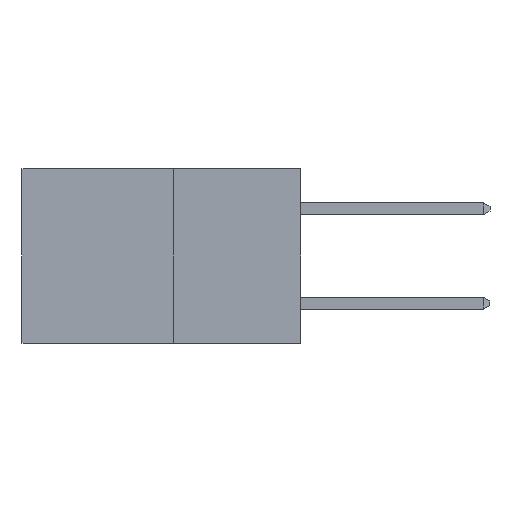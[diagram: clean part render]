
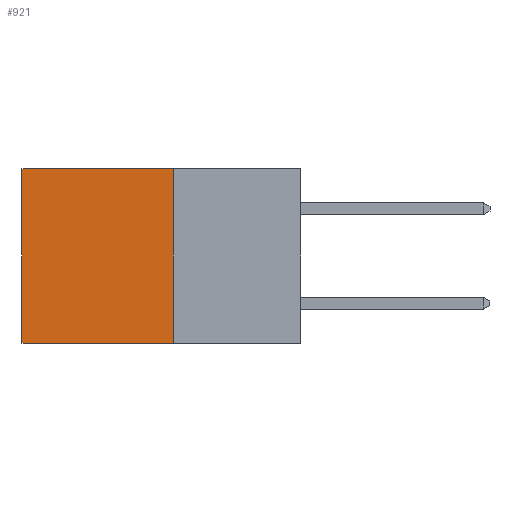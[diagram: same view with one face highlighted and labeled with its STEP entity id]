
A CAD part, left-side view. The second image highlights one B-rep face of the part: STEP entity #921.
In plain terms, the highlighted planar face has unit normal (-1, 0, 0).
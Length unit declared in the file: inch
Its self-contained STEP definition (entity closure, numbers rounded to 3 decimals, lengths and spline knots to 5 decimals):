
#343 = CARTESIAN_POINT ( 'NONE',  ( 0.277, 0.27, -0.37 ) ) ;
#373 = EDGE_LOOP ( 'NONE', ( #2014, #1810, #726, #1979 ) ) ;
#726 = ORIENTED_EDGE ( 'NONE', *, *, #4513, .F. ) ;
#759 = CARTESIAN_POINT ( 'NONE',  ( 0.277, 0.27, -0.37 ) ) ;
#921 = ADVANCED_FACE ( 'NONE', ( #6134 ), #6779, .F. ) ;
#927 = VERTEX_POINT ( 'NONE', #343 ) ;
#1200 = EDGE_CURVE ( 'NONE', #4449, #5701, #6830, .T. ) ;
#1810 = ORIENTED_EDGE ( 'NONE', *, *, #2150, .F. ) ;
#1979 = ORIENTED_EDGE ( 'NONE', *, *, #7679, .T. ) ;
#2014 = ORIENTED_EDGE ( 'NONE', *, *, #1200, .T. ) ;
#2150 = EDGE_CURVE ( 'NONE', #927, #5701, #4479, .T. ) ;
#3275 = VECTOR ( 'NONE', #7801, 39.37008 ) ;
#3278 = CARTESIAN_POINT ( 'NONE',  ( 0.277, 0.59, 0. ) ) ;
#3929 = VECTOR ( 'NONE', #7416, 39.37008 ) ;
#4286 = VECTOR ( 'NONE', #6316, 39.37008 ) ;
#4449 = VERTEX_POINT ( 'NONE', #3278 ) ;
#4478 = LINE ( 'NONE', #6309, #4286 ) ;
#4479 = LINE ( 'NONE', #5652, #3275 ) ;
#4513 = EDGE_CURVE ( 'NONE', #7478, #927, #4478, .T. ) ;
#4725 = DIRECTION ( 'NONE',  ( 1., 0., 0. ) ) ;
#4797 = VECTOR ( 'NONE', #7681, 39.37008 ) ;
#4952 = CARTESIAN_POINT ( 'NONE',  ( 0.277, 0.27, 0. ) ) ;
#5436 = DIRECTION ( 'NONE',  ( 0., 0., -1. ) ) ;
#5652 = CARTESIAN_POINT ( 'NONE',  ( 0.277, 0.27, -0.37 ) ) ;
#5701 = VERTEX_POINT ( 'NONE', #6427 ) ;
#6134 = FACE_OUTER_BOUND ( 'NONE', #373, .T. ) ;
#6309 = CARTESIAN_POINT ( 'NONE',  ( 0.277, 0.27, -0.37 ) ) ;
#6316 = DIRECTION ( 'NONE',  ( 0., 0., -1. ) ) ;
#6351 = LINE ( 'NONE', #7615, #4797 ) ;
#6427 = CARTESIAN_POINT ( 'NONE',  ( 0.277, 0.59, -0.37 ) ) ;
#6779 = PLANE ( 'NONE',  #7585 ) ;
#6830 = LINE ( 'NONE', #6902, #3929 ) ;
#6902 = CARTESIAN_POINT ( 'NONE',  ( 0.277, 0.59, -0.37 ) ) ;
#7416 = DIRECTION ( 'NONE',  ( 0., 0., -1. ) ) ;
#7478 = VERTEX_POINT ( 'NONE', #4952 ) ;
#7585 = AXIS2_PLACEMENT_3D ( 'NONE', #759, #4725, #5436 ) ;
#7615 = CARTESIAN_POINT ( 'NONE',  ( 0.277, 0.27, 0. ) ) ;
#7679 = EDGE_CURVE ( 'NONE', #7478, #4449, #6351, .T. ) ;
#7681 = DIRECTION ( 'NONE',  ( 0., 1., 0. ) ) ;
#7801 = DIRECTION ( 'NONE',  ( 0., 1., 0. ) ) ;
